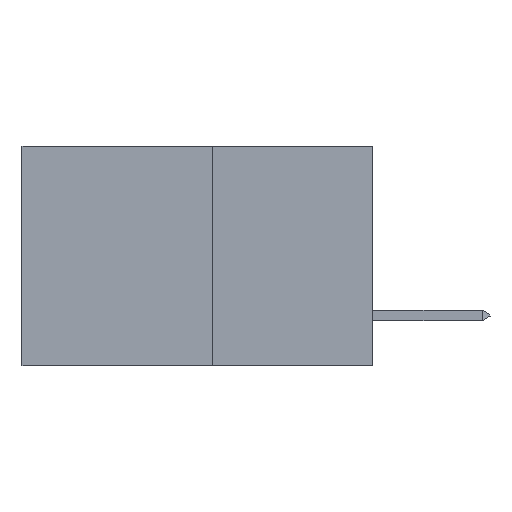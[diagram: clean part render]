
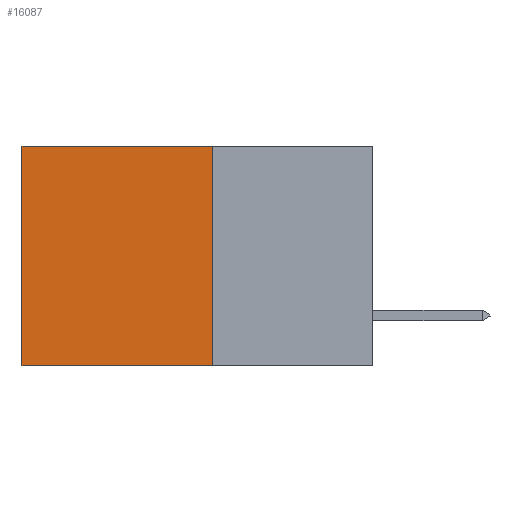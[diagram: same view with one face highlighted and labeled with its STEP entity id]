
A CAD part, left-side view. The second image highlights one B-rep face of the part: STEP entity #16087.
In plain terms, the highlighted planar face has unit normal (-1, 0, 0).
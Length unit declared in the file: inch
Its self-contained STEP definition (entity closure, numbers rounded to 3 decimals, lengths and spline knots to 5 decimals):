
#1314 = VERTEX_POINT ( 'NONE', #17744 ) ;
#1681 = CARTESIAN_POINT ( 'NONE',  ( 0.277, 0.27, -0.37 ) ) ;
#2446 = CARTESIAN_POINT ( 'NONE',  ( 0.277, 0.59, -0.37 ) ) ;
#2664 = LINE ( 'NONE', #8845, #17270 ) ;
#4598 = DIRECTION ( 'NONE',  ( 0., 0., -1. ) ) ;
#5467 = DIRECTION ( 'NONE',  ( 0., 1., 0. ) ) ;
#5816 = ORIENTED_EDGE ( 'NONE', *, *, #19564, .F. ) ;
#6441 = LINE ( 'NONE', #1681, #24131 ) ;
#6731 = DIRECTION ( 'NONE',  ( 0., 1., 0. ) ) ;
#8608 = AXIS2_PLACEMENT_3D ( 'NONE', #19697, #16039, #4598 ) ;
#8698 = FACE_OUTER_BOUND ( 'NONE', #14799, .T. ) ;
#8845 = CARTESIAN_POINT ( 'NONE',  ( 0.277, 0.27, -0.37 ) ) ;
#9240 = ORIENTED_EDGE ( 'NONE', *, *, #23512, .F. ) ;
#9313 = CARTESIAN_POINT ( 'NONE',  ( 0.277, 0.59, 0. ) ) ;
#9407 = EDGE_CURVE ( 'NONE', #20607, #12571, #16474, .T. ) ;
#10492 = CARTESIAN_POINT ( 'NONE',  ( 0.277, 0.27, 0. ) ) ;
#10507 = LINE ( 'NONE', #2446, #15628 ) ;
#11284 = ORIENTED_EDGE ( 'NONE', *, *, #9407, .T. ) ;
#12571 = VERTEX_POINT ( 'NONE', #9313 ) ;
#13084 = VERTEX_POINT ( 'NONE', #14758 ) ;
#13907 = DIRECTION ( 'NONE',  ( 0., 0., -1. ) ) ;
#14143 = PLANE ( 'NONE',  #8608 ) ;
#14694 = ORIENTED_EDGE ( 'NONE', *, *, #16005, .T. ) ;
#14758 = CARTESIAN_POINT ( 'NONE',  ( 0.277, 0.27, -0.37 ) ) ;
#14799 = EDGE_LOOP ( 'NONE', ( #14694, #9240, #5816, #11284 ) ) ;
#15133 = CARTESIAN_POINT ( 'NONE',  ( 0.277, 0.27, 0. ) ) ;
#15628 = VECTOR ( 'NONE', #13907, 39.37008 ) ;
#16005 = EDGE_CURVE ( 'NONE', #12571, #1314, #10507, .T. ) ;
#16039 = DIRECTION ( 'NONE',  ( 1., 0., 0. ) ) ;
#16087 = ADVANCED_FACE ( 'NONE', ( #8698 ), #14143, .F. ) ;
#16474 = LINE ( 'NONE', #10492, #21961 ) ;
#16563 = DIRECTION ( 'NONE',  ( 0., 0., -1. ) ) ;
#17270 = VECTOR ( 'NONE', #16563, 39.37008 ) ;
#17744 = CARTESIAN_POINT ( 'NONE',  ( 0.277, 0.59, -0.37 ) ) ;
#19564 = EDGE_CURVE ( 'NONE', #20607, #13084, #2664, .T. ) ;
#19697 = CARTESIAN_POINT ( 'NONE',  ( 0.277, 0.27, -0.37 ) ) ;
#20607 = VERTEX_POINT ( 'NONE', #15133 ) ;
#21961 = VECTOR ( 'NONE', #6731, 39.37008 ) ;
#23512 = EDGE_CURVE ( 'NONE', #13084, #1314, #6441, .T. ) ;
#24131 = VECTOR ( 'NONE', #5467, 39.37008 ) ;
